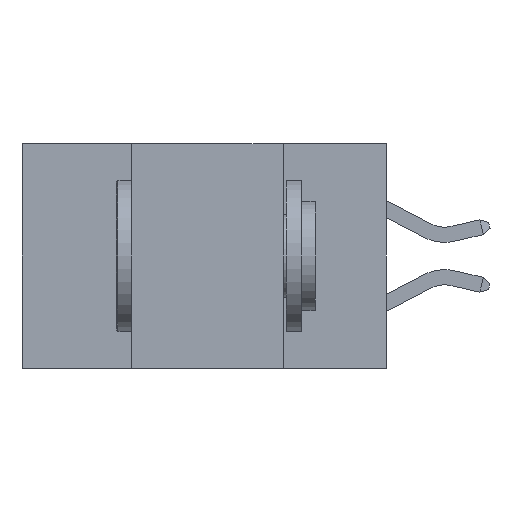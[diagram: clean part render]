
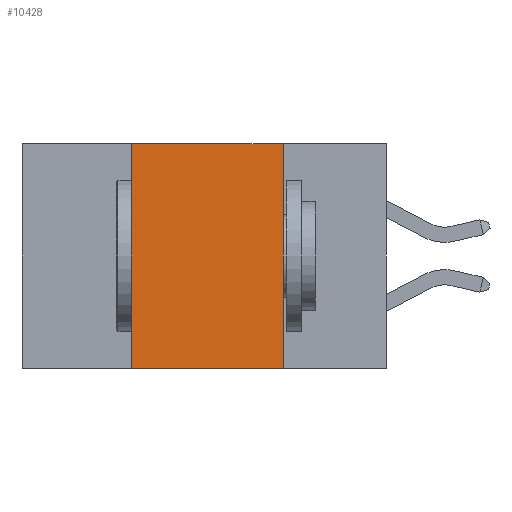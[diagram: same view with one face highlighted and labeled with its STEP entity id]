
A CAD part, left-side view. The second image highlights one B-rep face of the part: STEP entity #10428.
In plain terms, the highlighted planar face has unit normal (-1, 0, 0).
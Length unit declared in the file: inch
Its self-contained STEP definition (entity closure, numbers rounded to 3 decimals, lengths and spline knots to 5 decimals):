
#370 = ORIENTED_EDGE ( 'NONE', *, *, #17607, .T. ) ;
#895 = EDGE_LOOP ( 'NONE', ( #8589, #6101, #2586, #370 ) ) ;
#898 = VERTEX_POINT ( 'NONE', #8327 ) ;
#1078 = VECTOR ( 'NONE', #5882, 39.37008 ) ;
#1238 = EDGE_CURVE ( 'NONE', #6872, #898, #10901, .T. ) ;
#1977 = VERTEX_POINT ( 'NONE', #5396 ) ;
#2084 = FACE_OUTER_BOUND ( 'NONE', #895, .T. ) ;
#2153 = DIRECTION ( 'NONE',  ( 0., 0., -1. ) ) ;
#2312 = AXIS2_PLACEMENT_3D ( 'NONE', #9287, #10707, #2153 ) ;
#2586 = ORIENTED_EDGE ( 'NONE', *, *, #4550, .F. ) ;
#3061 = LINE ( 'NONE', #11078, #10182 ) ;
#3245 = VECTOR ( 'NONE', #13169, 39.37008 ) ;
#4193 = VERTEX_POINT ( 'NONE', #7661 ) ;
#4431 = CARTESIAN_POINT ( 'NONE',  ( 0., 0.6, -0.37 ) ) ;
#4550 = EDGE_CURVE ( 'NONE', #4193, #6872, #7084, .T. ) ;
#5396 = CARTESIAN_POINT ( 'NONE',  ( 0., 0.17, -0.37 ) ) ;
#5882 = DIRECTION ( 'NONE',  ( 0., -1., 0. ) ) ;
#6101 = ORIENTED_EDGE ( 'NONE', *, *, #1238, .F. ) ;
#6872 = VERTEX_POINT ( 'NONE', #15738 ) ;
#7084 = LINE ( 'NONE', #16189, #3245 ) ;
#7098 = DIRECTION ( 'NONE',  ( 0., -1., 0. ) ) ;
#7661 = CARTESIAN_POINT ( 'NONE',  ( 0., 0.42, -0.37 ) ) ;
#7896 = CARTESIAN_POINT ( 'NONE',  ( 0., 0.6, 0. ) ) ;
#8288 = DIRECTION ( 'NONE',  ( 0., 0., -1. ) ) ;
#8327 = CARTESIAN_POINT ( 'NONE',  ( 0., 0.17, 0. ) ) ;
#8589 = ORIENTED_EDGE ( 'NONE', *, *, #15043, .F. ) ;
#9287 = CARTESIAN_POINT ( 'NONE',  ( 0., 0.6, 0. ) ) ;
#10182 = VECTOR ( 'NONE', #8288, 39.37008 ) ;
#10428 = ADVANCED_FACE ( 'NONE', ( #2084 ), #17438, .F. ) ;
#10457 = VECTOR ( 'NONE', #7098, 39.37008 ) ;
#10707 = DIRECTION ( 'NONE',  ( 1., 0., 0. ) ) ;
#10901 = LINE ( 'NONE', #7896, #10457 ) ;
#11078 = CARTESIAN_POINT ( 'NONE',  ( 0., 0.17, 0. ) ) ;
#13169 = DIRECTION ( 'NONE',  ( 0., 0., 1. ) ) ;
#15043 = EDGE_CURVE ( 'NONE', #898, #1977, #3061, .T. ) ;
#15586 = LINE ( 'NONE', #4431, #1078 ) ;
#15738 = CARTESIAN_POINT ( 'NONE',  ( 0., 0.42, 0. ) ) ;
#16189 = CARTESIAN_POINT ( 'NONE',  ( 0., 0.42, 0. ) ) ;
#17438 = PLANE ( 'NONE',  #2312 ) ;
#17607 = EDGE_CURVE ( 'NONE', #4193, #1977, #15586, .T. ) ;
